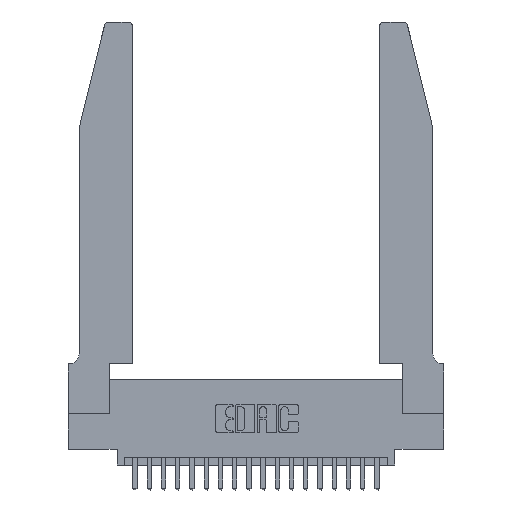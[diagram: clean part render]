
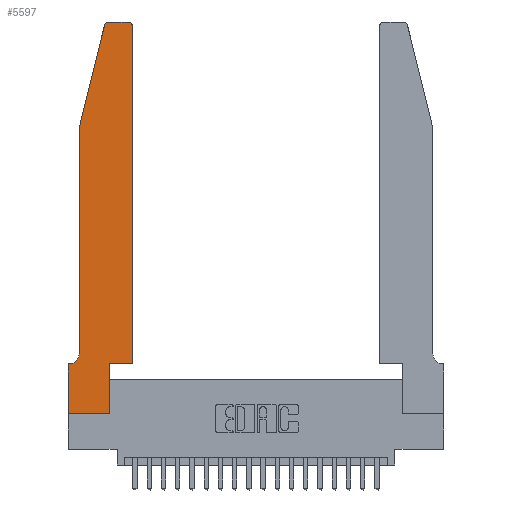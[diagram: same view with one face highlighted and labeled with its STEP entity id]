
A CAD part, top view. The second image highlights one B-rep face of the part: STEP entity #5597.
In plain terms, the highlighted planar face has unit normal (0, 0, 1).
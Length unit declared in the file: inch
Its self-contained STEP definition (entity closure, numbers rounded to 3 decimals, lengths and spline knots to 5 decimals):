
#64 = VECTOR ( 'NONE', #21082, 39.37008 ) ;
#416 = CARTESIAN_POINT ( 'NONE',  ( 0.4505, 0.35, 0.37 ) ) ;
#769 = ORIENTED_EDGE ( 'NONE', *, *, #11976, .T. ) ;
#918 = CARTESIAN_POINT ( 'NONE',  ( 0.0755, 2., 0.37 ) ) ;
#1366 = EDGE_CURVE ( 'NONE', #15446, #19010, #19221, .T. ) ;
#1532 = DIRECTION ( 'NONE',  ( 1., 0., 0. ) ) ;
#2089 = DIRECTION ( 'NONE',  ( 0., 0., 1. ) ) ;
#2504 = CIRCLE ( 'NONE', #14895, 0.03 ) ;
#2853 = EDGE_CURVE ( 'NONE', #16636, #16393, #2504, .T. ) ;
#2875 = LINE ( 'NONE', #3269, #15476 ) ;
#3269 = CARTESIAN_POINT ( 'NONE',  ( 0., 0., 0.37 ) ) ;
#3422 = EDGE_CURVE ( 'NONE', #11219, #7464, #12990, .T. ) ;
#4400 = CARTESIAN_POINT ( 'NONE',  ( 0.0055, 0.42, 0.37 ) ) ;
#4600 = VERTEX_POINT ( 'NONE', #10360 ) ;
#4898 = FACE_OUTER_BOUND ( 'NONE', #17308, .T. ) ;
#5035 = CARTESIAN_POINT ( 'NONE',  ( 0., 0.35, 0.37 ) ) ;
#5137 = ORIENTED_EDGE ( 'NONE', *, *, #20904, .T. ) ;
#5167 = VERTEX_POINT ( 'NONE', #416 ) ;
#5597 = ADVANCED_FACE ( 'NONE', ( #4898 ), #16957, .T. ) ;
#5631 = CIRCLE ( 'NONE', #10214, 0.03 ) ;
#6146 = DIRECTION ( 'NONE',  ( -1., 0., 0. ) ) ;
#6162 = ORIENTED_EDGE ( 'NONE', *, *, #21105, .T. ) ;
#6327 = CARTESIAN_POINT ( 'NONE',  ( 0.4205, 2.75, 0.37 ) ) ;
#6651 = EDGE_CURVE ( 'NONE', #9266, #12955, #12336, .T. ) ;
#6968 = VECTOR ( 'NONE', #18554, 39.37008 ) ;
#7129 = CARTESIAN_POINT ( 'NONE',  ( 0., 0., 0.37 ) ) ;
#7214 = EDGE_CURVE ( 'NONE', #12955, #16919, #10736, .T. ) ;
#7360 = ORIENTED_EDGE ( 'NONE', *, *, #3422, .T. ) ;
#7464 = VERTEX_POINT ( 'NONE', #12271 ) ;
#7607 = ORIENTED_EDGE ( 'NONE', *, *, #14386, .T. ) ;
#7665 = AXIS2_PLACEMENT_3D ( 'NONE', #5035, #11904, #1532 ) ;
#7857 = CARTESIAN_POINT ( 'NONE',  ( 0., 0., 0.37 ) ) ;
#7931 = DIRECTION ( 'NONE',  ( -0.239, -0.971, 0. ) ) ;
#8097 = CARTESIAN_POINT ( 'NONE',  ( 0.4505, 2.72, 0.37 ) ) ;
#8195 = CARTESIAN_POINT ( 'NONE',  ( 0.0755, 2., 0.37 ) ) ;
#8360 = LINE ( 'NONE', #19463, #21421 ) ;
#8661 = CIRCLE ( 'NONE', #10960, 0.07 ) ;
#8790 = CARTESIAN_POINT ( 'NONE',  ( 0.2865, 0.35, 0.37 ) ) ;
#9080 = EDGE_CURVE ( 'NONE', #5167, #16636, #11509, .T. ) ;
#9180 = CARTESIAN_POINT ( 'NONE',  ( 0.2865, 0.35, 0.37 ) ) ;
#9266 = VERTEX_POINT ( 'NONE', #13874 ) ;
#9592 = DIRECTION ( 'NONE',  ( 0., 0., 1. ) ) ;
#10154 = VECTOR ( 'NONE', #19442, 39.37008 ) ;
#10214 = AXIS2_PLACEMENT_3D ( 'NONE', #19786, #9592, #21480 ) ;
#10360 = CARTESIAN_POINT ( 'NONE',  ( 0.284, 2.75, 0.37 ) ) ;
#10556 = CARTESIAN_POINT ( 'NONE',  ( 0.0755, 0.42, 0.37 ) ) ;
#10736 = LINE ( 'NONE', #8195, #18687 ) ;
#10960 = AXIS2_PLACEMENT_3D ( 'NONE', #4400, #16329, #6146 ) ;
#11219 = VERTEX_POINT ( 'NONE', #7857 ) ;
#11509 = LINE ( 'NONE', #18469, #6968 ) ;
#11856 = DIRECTION ( 'NONE',  ( 0., -1., 0. ) ) ;
#11904 = DIRECTION ( 'NONE',  ( 0., 0., 1. ) ) ;
#11919 = DIRECTION ( 'NONE',  ( 1., 0., 0. ) ) ;
#11976 = EDGE_CURVE ( 'NONE', #20067, #5167, #14300, .T. ) ;
#12271 = CARTESIAN_POINT ( 'NONE',  ( 0.2865, 0., 0.37 ) ) ;
#12336 = LINE ( 'NONE', #918, #17389 ) ;
#12426 = CARTESIAN_POINT ( 'NONE',  ( 0.4205, 2.72, 0.37 ) ) ;
#12955 = VERTEX_POINT ( 'NONE', #19435 ) ;
#12990 = LINE ( 'NONE', #7129, #22051 ) ;
#13075 = EDGE_CURVE ( 'NONE', #16919, #15446, #8661, .T. ) ;
#13269 = ORIENTED_EDGE ( 'NONE', *, *, #7214, .T. ) ;
#13359 = CARTESIAN_POINT ( 'NONE',  ( 0., 0.35, 0.37 ) ) ;
#13409 = ORIENTED_EDGE ( 'NONE', *, *, #1366, .T. ) ;
#13420 = LINE ( 'NONE', #9180, #64 ) ;
#13874 = CARTESIAN_POINT ( 'NONE',  ( 0.25487, 2.72718, 0.37 ) ) ;
#14080 = ORIENTED_EDGE ( 'NONE', *, *, #9080, .T. ) ;
#14142 = DIRECTION ( 'NONE',  ( 1., 0., 0. ) ) ;
#14227 = ORIENTED_EDGE ( 'NONE', *, *, #6651, .T. ) ;
#14300 = LINE ( 'NONE', #22137, #18270 ) ;
#14346 = EDGE_CURVE ( 'NONE', #7464, #20067, #13420, .T. ) ;
#14386 = EDGE_CURVE ( 'NONE', #16393, #4600, #8360, .T. ) ;
#14895 = AXIS2_PLACEMENT_3D ( 'NONE', #12426, #2089, #14142 ) ;
#14959 = DIRECTION ( 'NONE',  ( 0., -1., 0. ) ) ;
#15446 = VERTEX_POINT ( 'NONE', #21036 ) ;
#15476 = VECTOR ( 'NONE', #11856, 39.37008 ) ;
#16016 = ORIENTED_EDGE ( 'NONE', *, *, #2853, .T. ) ;
#16329 = DIRECTION ( 'NONE',  ( 0., 0., -1. ) ) ;
#16393 = VERTEX_POINT ( 'NONE', #6327 ) ;
#16636 = VERTEX_POINT ( 'NONE', #8097 ) ;
#16919 = VERTEX_POINT ( 'NONE', #10556 ) ;
#16957 = PLANE ( 'NONE',  #7665 ) ;
#17300 = DIRECTION ( 'NONE',  ( 1., 0., 0. ) ) ;
#17308 = EDGE_LOOP ( 'NONE', ( #7607, #5137, #14227, #13269, #21204, #13409, #6162, #7360, #20982, #769, #14080, #16016 ) ) ;
#17389 = VECTOR ( 'NONE', #7931, 39.37008 ) ;
#17737 = CARTESIAN_POINT ( 'NONE',  ( 0.0755, 0.35, 0.37 ) ) ;
#18270 = VECTOR ( 'NONE', #11919, 39.37008 ) ;
#18469 = CARTESIAN_POINT ( 'NONE',  ( 0.4505, 0.35, 0.37 ) ) ;
#18554 = DIRECTION ( 'NONE',  ( 0., 1., 0. ) ) ;
#18687 = VECTOR ( 'NONE', #14959, 39.37008 ) ;
#19010 = VERTEX_POINT ( 'NONE', #13359 ) ;
#19221 = LINE ( 'NONE', #17737, #10154 ) ;
#19435 = CARTESIAN_POINT ( 'NONE',  ( 0.0755, 2., 0.37 ) ) ;
#19442 = DIRECTION ( 'NONE',  ( -1., 0., 0. ) ) ;
#19463 = CARTESIAN_POINT ( 'NONE',  ( 0.2605, 2.75, 0.37 ) ) ;
#19786 = CARTESIAN_POINT ( 'NONE',  ( 0.284, 2.72, 0.37 ) ) ;
#20067 = VERTEX_POINT ( 'NONE', #8790 ) ;
#20904 = EDGE_CURVE ( 'NONE', #4600, #9266, #5631, .T. ) ;
#20982 = ORIENTED_EDGE ( 'NONE', *, *, #14346, .T. ) ;
#21036 = CARTESIAN_POINT ( 'NONE',  ( 0.0055, 0.35, 0.37 ) ) ;
#21082 = DIRECTION ( 'NONE',  ( 0., 1., 0. ) ) ;
#21105 = EDGE_CURVE ( 'NONE', #19010, #11219, #2875, .T. ) ;
#21152 = DIRECTION ( 'NONE',  ( -1., 0., 0. ) ) ;
#21204 = ORIENTED_EDGE ( 'NONE', *, *, #13075, .T. ) ;
#21421 = VECTOR ( 'NONE', #21152, 39.37008 ) ;
#21480 = DIRECTION ( 'NONE',  ( 1., 0., 0. ) ) ;
#22051 = VECTOR ( 'NONE', #17300, 39.37008 ) ;
#22137 = CARTESIAN_POINT ( 'NONE',  ( 0.4505, 0.35, 0.37 ) ) ;
